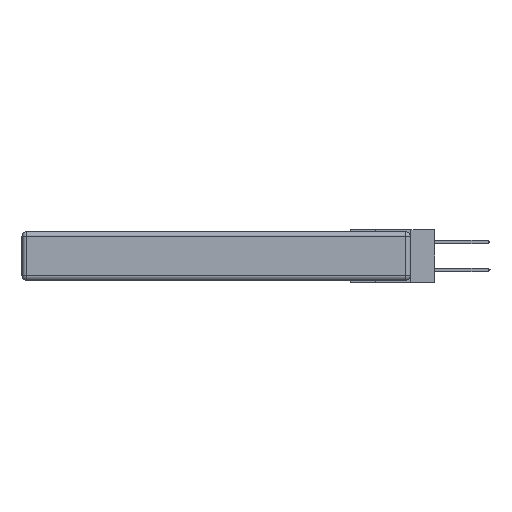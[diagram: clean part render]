
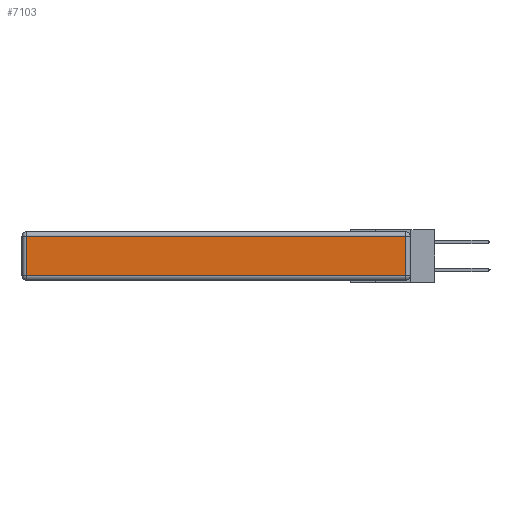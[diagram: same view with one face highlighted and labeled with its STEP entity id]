
A CAD part, left-side view. The second image highlights one B-rep face of the part: STEP entity #7103.
In plain terms, the highlighted planar face has unit normal (-1, 0, 0).
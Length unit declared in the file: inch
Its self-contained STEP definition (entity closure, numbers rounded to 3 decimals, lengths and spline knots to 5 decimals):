
#40 = LINE ( 'NONE', #17019, #11406 ) ;
#683 = DIRECTION ( 'NONE',  ( 0., -1., 0. ) ) ;
#686 = ORIENTED_EDGE ( 'NONE', *, *, #11743, .T. ) ;
#1249 = ORIENTED_EDGE ( 'NONE', *, *, #1499, .T. ) ;
#1278 = VERTEX_POINT ( 'NONE', #10315 ) ;
#1499 = EDGE_CURVE ( 'NONE', #7866, #12407, #13316, .T. ) ;
#2313 = DIRECTION ( 'NONE',  ( 0., 0., -1. ) ) ;
#3917 = CARTESIAN_POINT ( 'NONE',  ( 0., 0., -0.313 ) ) ;
#4835 = VECTOR ( 'NONE', #683, 39.37008 ) ;
#4924 = CARTESIAN_POINT ( 'NONE',  ( 0., 0.03, -0.343 ) ) ;
#6680 = LINE ( 'NONE', #3917, #4835 ) ;
#6755 = DIRECTION ( 'NONE',  ( -1., 0., 0. ) ) ;
#7103 = ADVANCED_FACE ( 'NONE', ( #10650 ), #10811, .T. ) ;
#7479 = EDGE_CURVE ( 'NONE', #12407, #1278, #17932, .T. ) ;
#7800 = EDGE_CURVE ( 'NONE', #10393, #7866, #6680, .T. ) ;
#7866 = VERTEX_POINT ( 'NONE', #17691 ) ;
#7884 = DIRECTION ( 'NONE',  ( 0., 0., 1. ) ) ;
#8129 = CARTESIAN_POINT ( 'NONE',  ( 0., 2.72, -0.313 ) ) ;
#8545 = VECTOR ( 'NONE', #7884, 39.37008 ) ;
#8576 = ORIENTED_EDGE ( 'NONE', *, *, #7479, .T. ) ;
#10148 = CARTESIAN_POINT ( 'NONE',  ( 0., 2.75, -0.03 ) ) ;
#10315 = CARTESIAN_POINT ( 'NONE',  ( 0., 2.72, -0.03 ) ) ;
#10380 = EDGE_LOOP ( 'NONE', ( #13500, #1249, #8576, #686 ) ) ;
#10393 = VERTEX_POINT ( 'NONE', #8129 ) ;
#10650 = FACE_OUTER_BOUND ( 'NONE', #10380, .T. ) ;
#10811 = PLANE ( 'NONE',  #13393 ) ;
#11364 = CARTESIAN_POINT ( 'NONE',  ( 0., 0., -0.343 ) ) ;
#11406 = VECTOR ( 'NONE', #2313, 39.37008 ) ;
#11743 = EDGE_CURVE ( 'NONE', #1278, #10393, #40, .T. ) ;
#12407 = VERTEX_POINT ( 'NONE', #16410 ) ;
#12891 = DIRECTION ( 'NONE',  ( 0., 0., 1. ) ) ;
#13316 = LINE ( 'NONE', #4924, #8545 ) ;
#13393 = AXIS2_PLACEMENT_3D ( 'NONE', #11364, #6755, #12891 ) ;
#13500 = ORIENTED_EDGE ( 'NONE', *, *, #7800, .T. ) ;
#13950 = VECTOR ( 'NONE', #16240, 39.37008 ) ;
#16240 = DIRECTION ( 'NONE',  ( 0., 1., 0. ) ) ;
#16410 = CARTESIAN_POINT ( 'NONE',  ( 0., 0.03, -0.03 ) ) ;
#17019 = CARTESIAN_POINT ( 'NONE',  ( 0., 2.72, -0.343 ) ) ;
#17691 = CARTESIAN_POINT ( 'NONE',  ( 0., 0.03, -0.313 ) ) ;
#17932 = LINE ( 'NONE', #10148, #13950 ) ;
